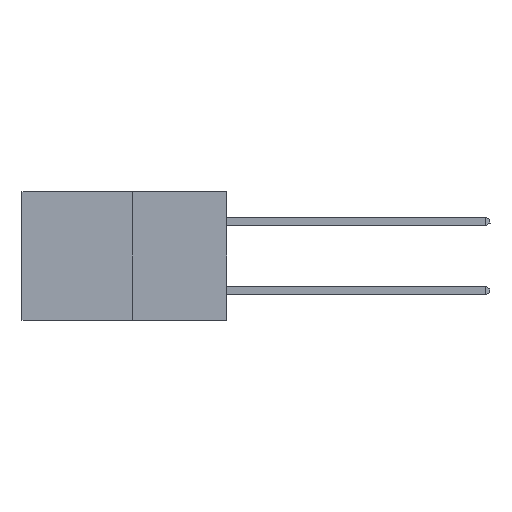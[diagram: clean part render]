
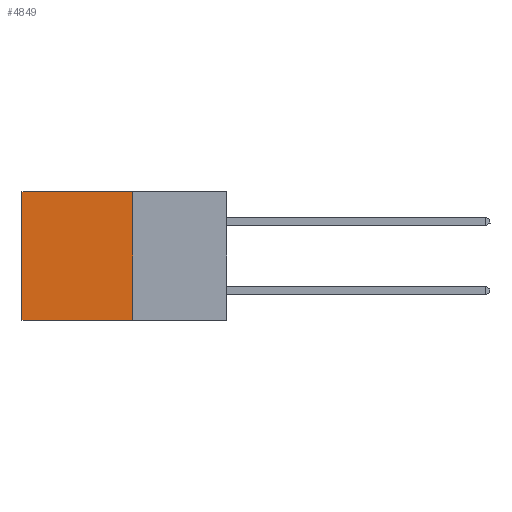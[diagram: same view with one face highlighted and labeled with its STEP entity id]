
A CAD part, left-side view. The second image highlights one B-rep face of the part: STEP entity #4849.
In plain terms, the highlighted planar face has unit normal (-1, 0, 0).
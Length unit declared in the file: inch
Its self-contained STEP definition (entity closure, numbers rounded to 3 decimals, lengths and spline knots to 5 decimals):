
#277 = VERTEX_POINT ( 'NONE', #8355 ) ;
#289 = FACE_OUTER_BOUND ( 'NONE', #1918, .T. ) ;
#500 = DIRECTION ( 'NONE',  ( 0., 1., 0. ) ) ;
#672 = CARTESIAN_POINT ( 'NONE',  ( 0.277, 0.27, -0.37 ) ) ;
#707 = ORIENTED_EDGE ( 'NONE', *, *, #7999, .T. ) ;
#754 = CARTESIAN_POINT ( 'NONE',  ( 0.277, 0.27, -0.37 ) ) ;
#1298 = EDGE_CURVE ( 'NONE', #3287, #4644, #8465, .T. ) ;
#1353 = ORIENTED_EDGE ( 'NONE', *, *, #1298, .F. ) ;
#1748 = PLANE ( 'NONE',  #3368 ) ;
#1805 = VECTOR ( 'NONE', #4386, 39.37008 ) ;
#1918 = EDGE_LOOP ( 'NONE', ( #2444, #1353, #6034, #707 ) ) ;
#2071 = CARTESIAN_POINT ( 'NONE',  ( 0.277, 0.59, -0.37 ) ) ;
#2103 = CARTESIAN_POINT ( 'NONE',  ( 0.277, 0.27, 0. ) ) ;
#2444 = ORIENTED_EDGE ( 'NONE', *, *, #6761, .T. ) ;
#2637 = DIRECTION ( 'NONE',  ( 1., 0., 0. ) ) ;
#3190 = VECTOR ( 'NONE', #9308, 39.37008 ) ;
#3287 = VERTEX_POINT ( 'NONE', #4351 ) ;
#3368 = AXIS2_PLACEMENT_3D ( 'NONE', #672, #2637, #8626 ) ;
#3526 = CARTESIAN_POINT ( 'NONE',  ( 0.277, 0.59, 0. ) ) ;
#4351 = CARTESIAN_POINT ( 'NONE',  ( 0.277, 0.27, -0.37 ) ) ;
#4386 = DIRECTION ( 'NONE',  ( 0., 1., 0. ) ) ;
#4644 = VERTEX_POINT ( 'NONE', #2071 ) ;
#4689 = LINE ( 'NONE', #2103, #6851 ) ;
#4849 = ADVANCED_FACE ( 'NONE', ( #289 ), #1748, .F. ) ;
#5201 = VECTOR ( 'NONE', #7077, 39.37008 ) ;
#6034 = ORIENTED_EDGE ( 'NONE', *, *, #6510, .F. ) ;
#6510 = EDGE_CURVE ( 'NONE', #277, #3287, #7418, .T. ) ;
#6761 = EDGE_CURVE ( 'NONE', #7502, #4644, #7307, .T. ) ;
#6851 = VECTOR ( 'NONE', #500, 39.37008 ) ;
#7063 = CARTESIAN_POINT ( 'NONE',  ( 0.277, 0.59, -0.37 ) ) ;
#7077 = DIRECTION ( 'NONE',  ( 0., 0., -1. ) ) ;
#7307 = LINE ( 'NONE', #7063, #5201 ) ;
#7418 = LINE ( 'NONE', #9297, #3190 ) ;
#7502 = VERTEX_POINT ( 'NONE', #3526 ) ;
#7999 = EDGE_CURVE ( 'NONE', #277, #7502, #4689, .T. ) ;
#8355 = CARTESIAN_POINT ( 'NONE',  ( 0.277, 0.27, 0. ) ) ;
#8465 = LINE ( 'NONE', #754, #1805 ) ;
#8626 = DIRECTION ( 'NONE',  ( 0., 0., -1. ) ) ;
#9297 = CARTESIAN_POINT ( 'NONE',  ( 0.277, 0.27, -0.37 ) ) ;
#9308 = DIRECTION ( 'NONE',  ( 0., 0., -1. ) ) ;
